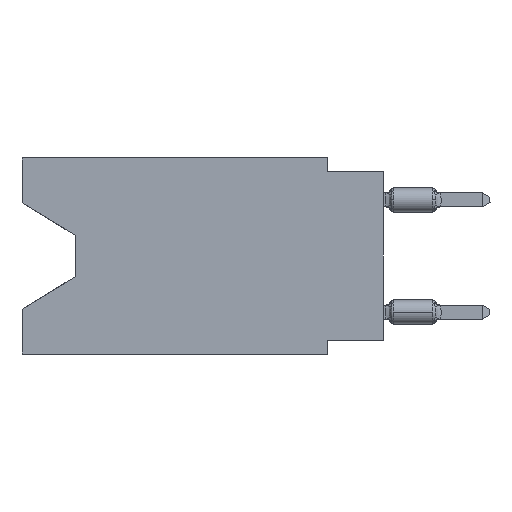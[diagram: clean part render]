
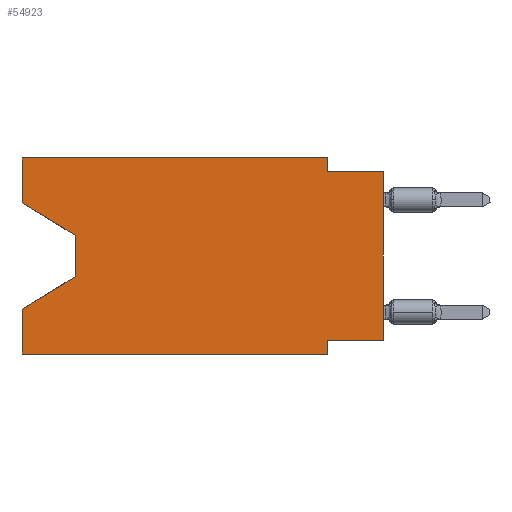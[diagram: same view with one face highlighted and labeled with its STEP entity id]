
A CAD part, left-side view. The second image highlights one B-rep face of the part: STEP entity #54923.
In plain terms, the highlighted planar face has unit normal (-1, 0, 0).
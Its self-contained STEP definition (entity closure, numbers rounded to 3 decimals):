
#716 = LINE ( 'NONE', #41313, #36382 ) ;
#1965 = DIRECTION ( 'NONE',  ( 0., -1., 0. ) ) ;
#2290 = VECTOR ( 'NONE', #39504, 1000. ) ;
#2757 = EDGE_CURVE ( 'NONE', #36177, #16401, #40906, .T. ) ;
#4086 = DIRECTION ( 'NONE',  ( 0., -1., 0. ) ) ;
#4304 = CARTESIAN_POINT ( 'NONE',  ( 0., 0., -8.255 ) ) ;
#4443 = EDGE_CURVE ( 'NONE', #59148, #58949, #58988, .T. ) ;
#6055 = CARTESIAN_POINT ( 'NONE',  ( 0., 2.54, -8.255 ) ) ;
#6753 = VERTEX_POINT ( 'NONE', #25342 ) ;
#6969 = EDGE_CURVE ( 'NONE', #26753, #16401, #716, .T. ) ;
#7805 = CARTESIAN_POINT ( 'NONE',  ( 0., 0., 0. ) ) ;
#7919 = LINE ( 'NONE', #8254, #10420 ) ;
#8254 = CARTESIAN_POINT ( 'NONE',  ( 0., 16.383, 0. ) ) ;
#9120 = LINE ( 'NONE', #50054, #40410 ) ;
#9376 = LINE ( 'NONE', #29678, #49245 ) ;
#10381 = LINE ( 'NONE', #30691, #57138 ) ;
#10420 = VECTOR ( 'NONE', #1965, 1000. ) ;
#10574 = DIRECTION ( 'NONE',  ( 1., 0., 0. ) ) ;
#10925 = DIRECTION ( 'NONE',  ( 0., 0., -1. ) ) ;
#11216 = DIRECTION ( 'NONE',  ( 0., 0., -1. ) ) ;
#11540 = FACE_OUTER_BOUND ( 'NONE', #35850, .T. ) ;
#14056 = CARTESIAN_POINT ( 'NONE',  ( 0., 0., -0.635 ) ) ;
#15750 = VERTEX_POINT ( 'NONE', #55384 ) ;
#15969 = CARTESIAN_POINT ( 'NONE',  ( 0., 13.97, -5.385 ) ) ;
#16235 = PLANE ( 'NONE',  #37872 ) ;
#16401 = VERTEX_POINT ( 'NONE', #26657 ) ;
#16746 = DIRECTION ( 'NONE',  ( 0., 0., 1. ) ) ;
#16897 = CARTESIAN_POINT ( 'NONE',  ( 0., 13.97, -5.385 ) ) ;
#18052 = ORIENTED_EDGE ( 'NONE', *, *, #18796, .T. ) ;
#18242 = EDGE_CURVE ( 'NONE', #15750, #50339, #52667, .T. ) ;
#18796 = EDGE_CURVE ( 'NONE', #15750, #55435, #9120, .T. ) ;
#21886 = DIRECTION ( 'NONE',  ( 0., 0.855, -0.519 ) ) ;
#22902 = EDGE_CURVE ( 'NONE', #26955, #36177, #9376, .T. ) ;
#23123 = DIRECTION ( 'NONE',  ( 0., 0., 1. ) ) ;
#24093 = LINE ( 'NONE', #33410, #58532 ) ;
#24987 = ORIENTED_EDGE ( 'NONE', *, *, #56195, .T. ) ;
#25078 = ORIENTED_EDGE ( 'NONE', *, *, #34573, .T. ) ;
#25342 = CARTESIAN_POINT ( 'NONE',  ( 0., 16.383, -6.852 ) ) ;
#25505 = CARTESIAN_POINT ( 'NONE',  ( 0., 16.383, 0. ) ) ;
#25786 = ORIENTED_EDGE ( 'NONE', *, *, #22902, .F. ) ;
#26657 = CARTESIAN_POINT ( 'NONE',  ( 0., 2.54, -8.89 ) ) ;
#26753 = VERTEX_POINT ( 'NONE', #47876 ) ;
#26955 = VERTEX_POINT ( 'NONE', #4304 ) ;
#27281 = EDGE_CURVE ( 'NONE', #26753, #6753, #39171, .T. ) ;
#27512 = VECTOR ( 'NONE', #10925, 1000. ) ;
#29678 = CARTESIAN_POINT ( 'NONE',  ( 0., 0., -8.255 ) ) ;
#30691 = CARTESIAN_POINT ( 'NONE',  ( 0., 13.97, -3.505 ) ) ;
#32810 = CARTESIAN_POINT ( 'NONE',  ( 0., 0., -0.635 ) ) ;
#33125 = ORIENTED_EDGE ( 'NONE', *, *, #6969, .T. ) ;
#33410 = CARTESIAN_POINT ( 'NONE',  ( 0., 2.54, 0. ) ) ;
#34573 = EDGE_CURVE ( 'NONE', #55435, #60889, #10381, .T. ) ;
#35850 = EDGE_LOOP ( 'NONE', ( #18052, #25078, #24987, #42918, #33125, #52948, #25786, #37445, #41255, #38656, #58840, #39730 ) ) ;
#36177 = VERTEX_POINT ( 'NONE', #6055 ) ;
#36382 = VECTOR ( 'NONE', #46295, 1000. ) ;
#37223 = CARTESIAN_POINT ( 'NONE',  ( 0., 2.54, 0. ) ) ;
#37445 = ORIENTED_EDGE ( 'NONE', *, *, #50053, .T. ) ;
#37872 = AXIS2_PLACEMENT_3D ( 'NONE', #46505, #10574, #11216 ) ;
#38656 = ORIENTED_EDGE ( 'NONE', *, *, #63272, .F. ) ;
#39171 = LINE ( 'NONE', #64116, #2290 ) ;
#39504 = DIRECTION ( 'NONE',  ( 0., 0., 1. ) ) ;
#39730 = ORIENTED_EDGE ( 'NONE', *, *, #18242, .F. ) ;
#39772 = CARTESIAN_POINT ( 'NONE',  ( 0., 16.383, 0. ) ) ;
#40410 = VECTOR ( 'NONE', #55367, 1000. ) ;
#40906 = LINE ( 'NONE', #50230, #27512 ) ;
#41255 = ORIENTED_EDGE ( 'NONE', *, *, #4443, .F. ) ;
#41313 = CARTESIAN_POINT ( 'NONE',  ( 0., 16.383, -8.89 ) ) ;
#41547 = LINE ( 'NONE', #16897, #51784 ) ;
#42918 = ORIENTED_EDGE ( 'NONE', *, *, #27281, .F. ) ;
#44194 = VECTOR ( 'NONE', #23123, 1000. ) ;
#46295 = DIRECTION ( 'NONE',  ( 0., -1., 0. ) ) ;
#46505 = CARTESIAN_POINT ( 'NONE',  ( 0., 16.383, 0. ) ) ;
#47688 = VECTOR ( 'NONE', #4086, 1000. ) ;
#47876 = CARTESIAN_POINT ( 'NONE',  ( 0., 16.383, -8.89 ) ) ;
#48521 = VERTEX_POINT ( 'NONE', #37223 ) ;
#48628 = CARTESIAN_POINT ( 'NONE',  ( 0., 13.97, -3.505 ) ) ;
#49245 = VECTOR ( 'NONE', #49976, 1000. ) ;
#49976 = DIRECTION ( 'NONE',  ( 0., 1., 0. ) ) ;
#50053 = EDGE_CURVE ( 'NONE', #26955, #58949, #60550, .T. ) ;
#50054 = CARTESIAN_POINT ( 'NONE',  ( 0., 16.383, -2.038 ) ) ;
#50230 = CARTESIAN_POINT ( 'NONE',  ( 0., 2.54, -8.89 ) ) ;
#50339 = VERTEX_POINT ( 'NONE', #39772 ) ;
#50999 = DIRECTION ( 'NONE',  ( 0., 0., -1. ) ) ;
#51784 = VECTOR ( 'NONE', #21886, 1000. ) ;
#52046 = VECTOR ( 'NONE', #16746, 1000. ) ;
#52667 = LINE ( 'NONE', #25505, #52046 ) ;
#52948 = ORIENTED_EDGE ( 'NONE', *, *, #2757, .F. ) ;
#53413 = CARTESIAN_POINT ( 'NONE',  ( 0., 2.54, -0.635 ) ) ;
#54923 = ADVANCED_FACE ( 'NONE', ( #11540 ), #16235, .F. ) ;
#55367 = DIRECTION ( 'NONE',  ( 0., -0.855, -0.519 ) ) ;
#55384 = CARTESIAN_POINT ( 'NONE',  ( 0., 16.383, -2.038 ) ) ;
#55435 = VERTEX_POINT ( 'NONE', #48628 ) ;
#56195 = EDGE_CURVE ( 'NONE', #60889, #6753, #41547, .T. ) ;
#57138 = VECTOR ( 'NONE', #50999, 1000. ) ;
#58532 = VECTOR ( 'NONE', #64684, 1000. ) ;
#58840 = ORIENTED_EDGE ( 'NONE', *, *, #60413, .F. ) ;
#58949 = VERTEX_POINT ( 'NONE', #32810 ) ;
#58988 = LINE ( 'NONE', #14056, #47688 ) ;
#59148 = VERTEX_POINT ( 'NONE', #53413 ) ;
#60413 = EDGE_CURVE ( 'NONE', #50339, #48521, #7919, .T. ) ;
#60550 = LINE ( 'NONE', #7805, #44194 ) ;
#60889 = VERTEX_POINT ( 'NONE', #15969 ) ;
#63272 = EDGE_CURVE ( 'NONE', #48521, #59148, #24093, .T. ) ;
#64116 = CARTESIAN_POINT ( 'NONE',  ( 0., 16.383, 0. ) ) ;
#64684 = DIRECTION ( 'NONE',  ( 0., 0., -1. ) ) ;
